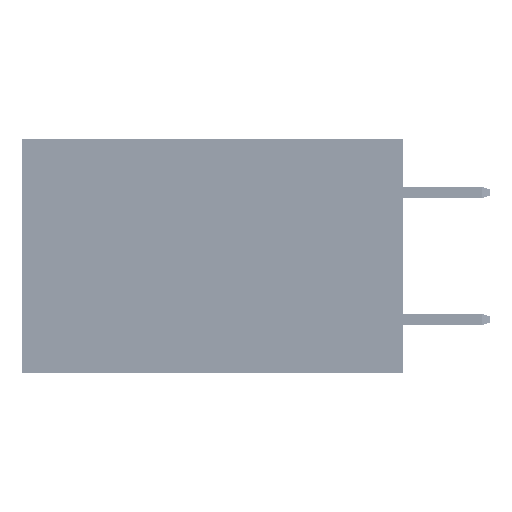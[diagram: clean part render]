
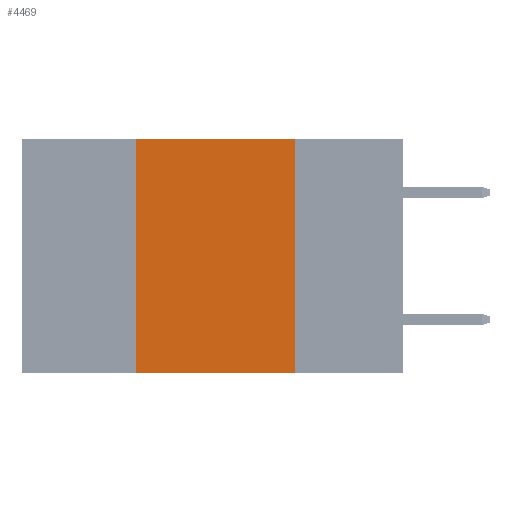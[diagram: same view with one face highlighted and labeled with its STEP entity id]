
A CAD part, left-side view. The second image highlights one B-rep face of the part: STEP entity #4469.
In plain terms, the highlighted planar face has unit normal (-1, 0, 0).
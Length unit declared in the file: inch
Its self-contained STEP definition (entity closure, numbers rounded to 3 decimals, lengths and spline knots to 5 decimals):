
#976 = CARTESIAN_POINT ( 'NONE',  ( 0., 0.6, -0.37 ) ) ;
#1900 = CARTESIAN_POINT ( 'NONE',  ( 0., 0.17, 0. ) ) ;
#3937 = ORIENTED_EDGE ( 'NONE', *, *, #11153, .T. ) ;
#4469 = ADVANCED_FACE ( 'NONE', ( #34972 ), #14231, .F. ) ;
#5448 = LINE ( 'NONE', #1900, #48333 ) ;
#6016 = CARTESIAN_POINT ( 'NONE',  ( 0., 0.17, 0. ) ) ;
#6064 = CARTESIAN_POINT ( 'NONE',  ( 0., 0.42, 0. ) ) ;
#7041 = VERTEX_POINT ( 'NONE', #21391 ) ;
#7050 = VECTOR ( 'NONE', #26702, 39.37008 ) ;
#8485 = LINE ( 'NONE', #28977, #28667 ) ;
#9422 = EDGE_CURVE ( 'NONE', #46248, #20865, #34346, .T. ) ;
#11153 = EDGE_CURVE ( 'NONE', #7041, #27943, #38347, .T. ) ;
#14231 = PLANE ( 'NONE',  #53112 ) ;
#14358 = ORIENTED_EDGE ( 'NONE', *, *, #46270, .F. ) ;
#17172 = CARTESIAN_POINT ( 'NONE',  ( 0., 0.6, 0. ) ) ;
#17793 = VECTOR ( 'NONE', #38615, 39.37008 ) ;
#18364 = EDGE_CURVE ( 'NONE', #20865, #27943, #5448, .T. ) ;
#18536 = DIRECTION ( 'NONE',  ( 0., 0., -1. ) ) ;
#20865 = VERTEX_POINT ( 'NONE', #6016 ) ;
#21391 = CARTESIAN_POINT ( 'NONE',  ( 0., 0.42, -0.37 ) ) ;
#22691 = DIRECTION ( 'NONE',  ( 1., 0., 0. ) ) ;
#26702 = DIRECTION ( 'NONE',  ( 0., -1., 0. ) ) ;
#27943 = VERTEX_POINT ( 'NONE', #41904 ) ;
#28667 = VECTOR ( 'NONE', #52969, 39.37008 ) ;
#28977 = CARTESIAN_POINT ( 'NONE',  ( 0., 0.42, 0. ) ) ;
#34346 = LINE ( 'NONE', #17172, #7050 ) ;
#34972 = FACE_OUTER_BOUND ( 'NONE', #40026, .T. ) ;
#35235 = DIRECTION ( 'NONE',  ( 0., 0., -1. ) ) ;
#38347 = LINE ( 'NONE', #976, #17793 ) ;
#38615 = DIRECTION ( 'NONE',  ( 0., -1., 0. ) ) ;
#39582 = CARTESIAN_POINT ( 'NONE',  ( 0., 0.6, 0. ) ) ;
#40026 = EDGE_LOOP ( 'NONE', ( #52810, #47452, #14358, #3937 ) ) ;
#41904 = CARTESIAN_POINT ( 'NONE',  ( 0., 0.17, -0.37 ) ) ;
#46248 = VERTEX_POINT ( 'NONE', #6064 ) ;
#46270 = EDGE_CURVE ( 'NONE', #7041, #46248, #8485, .T. ) ;
#47452 = ORIENTED_EDGE ( 'NONE', *, *, #9422, .F. ) ;
#48333 = VECTOR ( 'NONE', #18536, 39.37008 ) ;
#52810 = ORIENTED_EDGE ( 'NONE', *, *, #18364, .F. ) ;
#52969 = DIRECTION ( 'NONE',  ( 0., 0., 1. ) ) ;
#53112 = AXIS2_PLACEMENT_3D ( 'NONE', #39582, #22691, #35235 ) ;
